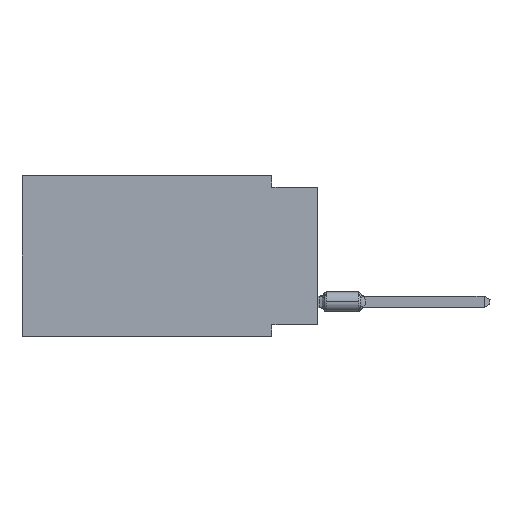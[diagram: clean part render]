
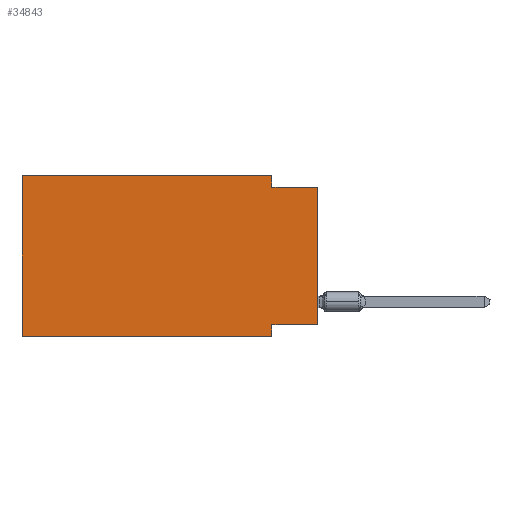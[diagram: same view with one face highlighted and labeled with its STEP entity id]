
A CAD part, left-side view. The second image highlights one B-rep face of the part: STEP entity #34843.
In plain terms, the highlighted planar face has unit normal (-1, 0, 0).
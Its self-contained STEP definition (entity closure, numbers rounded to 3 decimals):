
#2636 = LINE ( 'NONE', #28545, #33434 ) ;
#2845 = DIRECTION ( 'NONE',  ( 0., -1., 0. ) ) ;
#3972 = VECTOR ( 'NONE', #21614, 1000. ) ;
#4466 = VECTOR ( 'NONE', #30417, 1000. ) ;
#4482 = LINE ( 'NONE', #5041, #11056 ) ;
#5041 = CARTESIAN_POINT ( 'NONE',  ( 0., 0., 0. ) ) ;
#5325 = VERTEX_POINT ( 'NONE', #54550 ) ;
#7045 = VECTOR ( 'NONE', #14621, 1000. ) ;
#7118 = ORIENTED_EDGE ( 'NONE', *, *, #21617, .F. ) ;
#7957 = ORIENTED_EDGE ( 'NONE', *, *, #15225, .T. ) ;
#8218 = DIRECTION ( 'NONE',  ( 0., 0., 1. ) ) ;
#8385 = EDGE_CURVE ( 'NONE', #30194, #5325, #52940, .T. ) ;
#9118 = CARTESIAN_POINT ( 'NONE',  ( 0., 2.54, 0. ) ) ;
#11056 = VECTOR ( 'NONE', #34361, 1000. ) ;
#11312 = ORIENTED_EDGE ( 'NONE', *, *, #55525, .F. ) ;
#11631 = EDGE_CURVE ( 'NONE', #16573, #5325, #4482, .T. ) ;
#12161 = EDGE_LOOP ( 'NONE', ( #18555, #24646, #40362, #11312, #7118, #7957, #30188, #45061 ) ) ;
#14621 = DIRECTION ( 'NONE',  ( 0., 1., 0. ) ) ;
#15225 = EDGE_CURVE ( 'NONE', #26888, #16023, #41162, .T. ) ;
#15570 = VERTEX_POINT ( 'NONE', #9118 ) ;
#16023 = VERTEX_POINT ( 'NONE', #33592 ) ;
#16573 = VERTEX_POINT ( 'NONE', #42121 ) ;
#16870 = VECTOR ( 'NONE', #8218, 1000. ) ;
#17673 = LINE ( 'NONE', #43042, #3972 ) ;
#17843 = CARTESIAN_POINT ( 'NONE',  ( 0., 16.383, -8.89 ) ) ;
#17986 = LINE ( 'NONE', #23624, #25815 ) ;
#18509 = AXIS2_PLACEMENT_3D ( 'NONE', #49900, #28500, #41448 ) ;
#18555 = ORIENTED_EDGE ( 'NONE', *, *, #11631, .T. ) ;
#19160 = EDGE_CURVE ( 'NONE', #35243, #16023, #17986, .T. ) ;
#21614 = DIRECTION ( 'NONE',  ( 0., -1., 0. ) ) ;
#21617 = EDGE_CURVE ( 'NONE', #26888, #30775, #46808, .T. ) ;
#23624 = CARTESIAN_POINT ( 'NONE',  ( 0., 2.54, -8.89 ) ) ;
#24274 = PLANE ( 'NONE',  #18509 ) ;
#24646 = ORIENTED_EDGE ( 'NONE', *, *, #8385, .F. ) ;
#25672 = CARTESIAN_POINT ( 'NONE',  ( 0., 16.383, 0. ) ) ;
#25815 = VECTOR ( 'NONE', #26997, 1000. ) ;
#26888 = VERTEX_POINT ( 'NONE', #17843 ) ;
#26997 = DIRECTION ( 'NONE',  ( 0., 0., -1. ) ) ;
#28500 = DIRECTION ( 'NONE',  ( 1., 0., 0. ) ) ;
#28545 = CARTESIAN_POINT ( 'NONE',  ( 0., 2.54, 0. ) ) ;
#30188 = ORIENTED_EDGE ( 'NONE', *, *, #19160, .F. ) ;
#30194 = VERTEX_POINT ( 'NONE', #50744 ) ;
#30417 = DIRECTION ( 'NONE',  ( 0., -1., 0. ) ) ;
#30775 = VERTEX_POINT ( 'NONE', #47772 ) ;
#32724 = FACE_OUTER_BOUND ( 'NONE', #12161, .T. ) ;
#33434 = VECTOR ( 'NONE', #34162, 1000. ) ;
#33592 = CARTESIAN_POINT ( 'NONE',  ( 0., 2.54, -8.89 ) ) ;
#33816 = CARTESIAN_POINT ( 'NONE',  ( 0., 16.383, -8.89 ) ) ;
#34162 = DIRECTION ( 'NONE',  ( 0., 0., -1. ) ) ;
#34361 = DIRECTION ( 'NONE',  ( 0., 0., 1. ) ) ;
#34843 = ADVANCED_FACE ( 'NONE', ( #32724 ), #24274, .F. ) ;
#35243 = VERTEX_POINT ( 'NONE', #46569 ) ;
#38315 = LINE ( 'NONE', #55505, #7045 ) ;
#40362 = ORIENTED_EDGE ( 'NONE', *, *, #41862, .F. ) ;
#41162 = LINE ( 'NONE', #33816, #55079 ) ;
#41448 = DIRECTION ( 'NONE',  ( 0., 0., -1. ) ) ;
#41862 = EDGE_CURVE ( 'NONE', #15570, #30194, #2636, .T. ) ;
#42121 = CARTESIAN_POINT ( 'NONE',  ( 0., 0., -8.255 ) ) ;
#43042 = CARTESIAN_POINT ( 'NONE',  ( 0., 16.383, 0. ) ) ;
#45061 = ORIENTED_EDGE ( 'NONE', *, *, #50468, .F. ) ;
#46569 = CARTESIAN_POINT ( 'NONE',  ( 0., 2.54, -8.255 ) ) ;
#46808 = LINE ( 'NONE', #25672, #16870 ) ;
#47772 = CARTESIAN_POINT ( 'NONE',  ( 0., 16.383, 0. ) ) ;
#49900 = CARTESIAN_POINT ( 'NONE',  ( 0., 16.383, 0. ) ) ;
#50468 = EDGE_CURVE ( 'NONE', #16573, #35243, #38315, .T. ) ;
#50744 = CARTESIAN_POINT ( 'NONE',  ( 0., 2.54, -0.635 ) ) ;
#52099 = CARTESIAN_POINT ( 'NONE',  ( 0., 0., -0.635 ) ) ;
#52940 = LINE ( 'NONE', #52099, #4466 ) ;
#54550 = CARTESIAN_POINT ( 'NONE',  ( 0., 0., -0.635 ) ) ;
#55079 = VECTOR ( 'NONE', #2845, 1000. ) ;
#55505 = CARTESIAN_POINT ( 'NONE',  ( 0., 0., -8.255 ) ) ;
#55525 = EDGE_CURVE ( 'NONE', #30775, #15570, #17673, .T. ) ;
